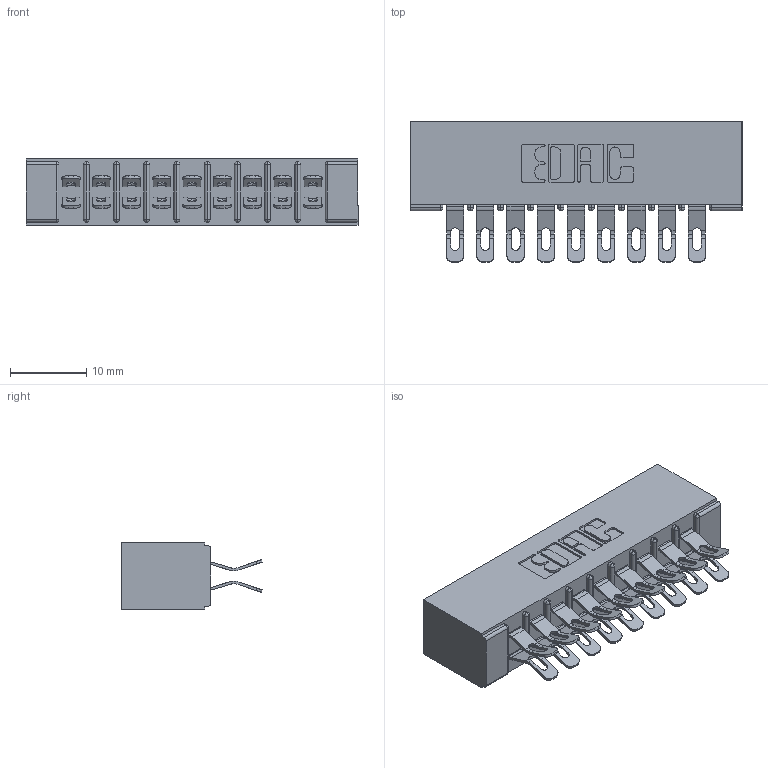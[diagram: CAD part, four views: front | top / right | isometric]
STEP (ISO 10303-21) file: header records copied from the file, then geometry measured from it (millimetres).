
FILE_DESCRIPTION (( 'STEP AP203' ), '1' );
FILE_NAME ('305-018-555-201.STEP', '2019-09-09T12:45:51', ( '' ), ( '' ), 'SwSTEP 2.0', 'SolidWorks 2016', '' );
FILE_SCHEMA (( 'CONFIG_CONTROL_DESIGN' ));
Length unit declared in the file: inch
Products named in the file (3): 305 Part_No Mounting; 305-290-001_555; 305-018-555-201
Assembly tree (19 placements, depth 2):
  305-018-555-201
    305 Part_No Mounting
    305-290-001_555  x18
Bounding box: 43.54 x 18.41 x 8.71 mm (x, y, z)
Volume: 2990.1 mm3; surface area: 5762.9 mm2
Topology: 19 solids, 19 shells, 1296 faces, 3847 edges, 2514 vertices
Faces by surface type: plane 640, cylinder 620, sphere 36
Entity records: 14108 total; most frequent: CARTESIAN_POINT 2351, ORIENTED_EDGE 2318, DIRECTION 2293, EDGE_CURVE 1159, LINE 885, VECTOR 885, VERTEX_POINT 746, AXIS2_PLACEMENT_3D 704
